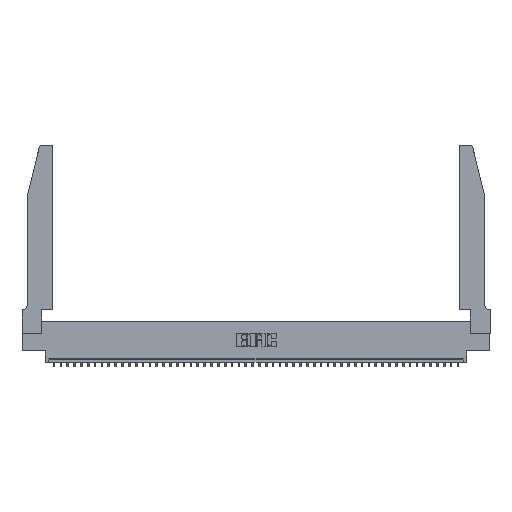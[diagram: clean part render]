
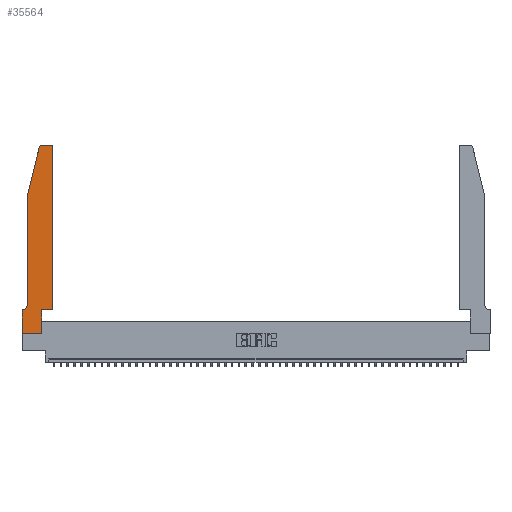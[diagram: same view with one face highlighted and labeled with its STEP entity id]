
A CAD part, top view. The second image highlights one B-rep face of the part: STEP entity #35564.
In plain terms, the highlighted planar face has unit normal (0, 0, 1).
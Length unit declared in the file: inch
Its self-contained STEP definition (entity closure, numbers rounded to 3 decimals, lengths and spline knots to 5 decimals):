
#1839 = CARTESIAN_POINT ( 'NONE',  ( 0.4505, 2.72, 0.37 ) ) ;
#1887 = DIRECTION ( 'NONE',  ( 1., 0., 0. ) ) ;
#2209 = VERTEX_POINT ( 'NONE', #33008 ) ;
#2397 = AXIS2_PLACEMENT_3D ( 'NONE', #25346, #14552, #6997 ) ;
#2660 = DIRECTION ( 'NONE',  ( 0., -1., 0. ) ) ;
#3910 = DIRECTION ( 'NONE',  ( 0., -1., 0. ) ) ;
#4577 = DIRECTION ( 'NONE',  ( 0., 1., 0. ) ) ;
#4760 = CARTESIAN_POINT ( 'NONE',  ( 0.2865, 0.35, 0.37 ) ) ;
#4791 = AXIS2_PLACEMENT_3D ( 'NONE', #44145, #21708, #29166 ) ;
#4852 = CARTESIAN_POINT ( 'NONE',  ( 0.2865, 0.35, 0.37 ) ) ;
#5420 = ORIENTED_EDGE ( 'NONE', *, *, #15437, .T. ) ;
#5461 = EDGE_CURVE ( 'NONE', #43064, #2209, #45747, .T. ) ;
#6198 = CIRCLE ( 'NONE', #37519, 0.03 ) ;
#6532 = CARTESIAN_POINT ( 'NONE',  ( 0.0755, 2., 0.37 ) ) ;
#6580 = LINE ( 'NONE', #20166, #33542 ) ;
#6997 = DIRECTION ( 'NONE',  ( 1., 0., 0. ) ) ;
#7316 = AXIS2_PLACEMENT_3D ( 'NONE', #16678, #38601, #20360 ) ;
#7540 = ORIENTED_EDGE ( 'NONE', *, *, #13173, .T. ) ;
#8031 = CARTESIAN_POINT ( 'NONE',  ( 0.0055, 0.35, 0.37 ) ) ;
#8186 = VECTOR ( 'NONE', #8944, 39.37008 ) ;
#8944 = DIRECTION ( 'NONE',  ( 1., 0., 0. ) ) ;
#11055 = EDGE_CURVE ( 'NONE', #25771, #43064, #26570, .T. ) ;
#12054 = VECTOR ( 'NONE', #23379, 39.37008 ) ;
#13173 = EDGE_CURVE ( 'NONE', #31391, #26869, #25869, .T. ) ;
#13547 = CARTESIAN_POINT ( 'NONE',  ( 0.284, 2.75, 0.37 ) ) ;
#13766 = ORIENTED_EDGE ( 'NONE', *, *, #5461, .T. ) ;
#13864 = CARTESIAN_POINT ( 'NONE',  ( 0.4505, 0.35, 0.37 ) ) ;
#14215 = VECTOR ( 'NONE', #4577, 39.37008 ) ;
#14552 = DIRECTION ( 'NONE',  ( 0., 0., 1. ) ) ;
#15160 = VECTOR ( 'NONE', #2660, 39.37008 ) ;
#15437 = EDGE_CURVE ( 'NONE', #26869, #45012, #25602, .T. ) ;
#15613 = ORIENTED_EDGE ( 'NONE', *, *, #32719, .T. ) ;
#16078 = DIRECTION ( 'NONE',  ( 1., 0., 0. ) ) ;
#16669 = ORIENTED_EDGE ( 'NONE', *, *, #11055, .T. ) ;
#16678 = CARTESIAN_POINT ( 'NONE',  ( 0., 0.35, 0.37 ) ) ;
#17177 = EDGE_CURVE ( 'NONE', #21071, #21904, #6580, .T. ) ;
#18057 = CARTESIAN_POINT ( 'NONE',  ( 0.4505, 0.35, 0.37 ) ) ;
#20040 = VECTOR ( 'NONE', #25182, 39.37008 ) ;
#20166 = CARTESIAN_POINT ( 'NONE',  ( 0.2605, 2.75, 0.37 ) ) ;
#20360 = DIRECTION ( 'NONE',  ( 1., 0., 0. ) ) ;
#20470 = LINE ( 'NONE', #4760, #14215 ) ;
#20518 = PLANE ( 'NONE',  #7316 ) ;
#21071 = VERTEX_POINT ( 'NONE', #40611 ) ;
#21300 = EDGE_CURVE ( 'NONE', #26277, #21071, #40802, .T. ) ;
#21496 = CARTESIAN_POINT ( 'NONE',  ( 0., 0., 0.37 ) ) ;
#21708 = DIRECTION ( 'NONE',  ( 0., 0., -1. ) ) ;
#21904 = VERTEX_POINT ( 'NONE', #13547 ) ;
#21989 = EDGE_CURVE ( 'NONE', #21904, #25771, #6198, .T. ) ;
#22930 = VECTOR ( 'NONE', #3910, 39.37008 ) ;
#23076 = VECTOR ( 'NONE', #23717, 39.37008 ) ;
#23379 = DIRECTION ( 'NONE',  ( -1., 0., 0. ) ) ;
#23558 = DIRECTION ( 'NONE',  ( -1., 0., 0. ) ) ;
#23619 = ORIENTED_EDGE ( 'NONE', *, *, #32257, .T. ) ;
#23717 = DIRECTION ( 'NONE',  ( -0.239, -0.971, 0. ) ) ;
#25182 = DIRECTION ( 'NONE',  ( 0., 1., 0. ) ) ;
#25346 = CARTESIAN_POINT ( 'NONE',  ( 0.4205, 2.72, 0.37 ) ) ;
#25602 = LINE ( 'NONE', #41126, #31373 ) ;
#25767 = EDGE_CURVE ( 'NONE', #45012, #26614, #20470, .T. ) ;
#25771 = VERTEX_POINT ( 'NONE', #30188 ) ;
#25869 = LINE ( 'NONE', #43743, #22930 ) ;
#26277 = VERTEX_POINT ( 'NONE', #1839 ) ;
#26570 = LINE ( 'NONE', #34330, #23076 ) ;
#26614 = VERTEX_POINT ( 'NONE', #4852 ) ;
#26829 = VERTEX_POINT ( 'NONE', #13864 ) ;
#26869 = VERTEX_POINT ( 'NONE', #21496 ) ;
#28531 = EDGE_CURVE ( 'NONE', #26614, #26829, #40473, .T. ) ;
#29166 = DIRECTION ( 'NONE',  ( -1., 0., 0. ) ) ;
#29934 = CARTESIAN_POINT ( 'NONE',  ( 0., 0.35, 0.37 ) ) ;
#30188 = CARTESIAN_POINT ( 'NONE',  ( 0.25487, 2.72718, 0.37 ) ) ;
#30238 = EDGE_LOOP ( 'NONE', ( #34583, #45160, #16669, #13766, #40182, #23619, #7540, #5420, #35904, #35687, #15613, #46600 ) ) ;
#30727 = CARTESIAN_POINT ( 'NONE',  ( 0.284, 2.72, 0.37 ) ) ;
#31373 = VECTOR ( 'NONE', #1887, 39.37008 ) ;
#31391 = VERTEX_POINT ( 'NONE', #29934 ) ;
#32257 = EDGE_CURVE ( 'NONE', #32406, #31391, #43799, .T. ) ;
#32406 = VERTEX_POINT ( 'NONE', #8031 ) ;
#32516 = CIRCLE ( 'NONE', #4791, 0.07 ) ;
#32719 = EDGE_CURVE ( 'NONE', #26829, #26277, #34463, .T. ) ;
#33008 = CARTESIAN_POINT ( 'NONE',  ( 0.0755, 0.42, 0.37 ) ) ;
#33542 = VECTOR ( 'NONE', #23558, 39.37008 ) ;
#34330 = CARTESIAN_POINT ( 'NONE',  ( 0.0755, 2., 0.37 ) ) ;
#34463 = LINE ( 'NONE', #18057, #20040 ) ;
#34583 = ORIENTED_EDGE ( 'NONE', *, *, #17177, .T. ) ;
#35564 = ADVANCED_FACE ( 'NONE', ( #46942 ), #20518, .T. ) ;
#35687 = ORIENTED_EDGE ( 'NONE', *, *, #28531, .T. ) ;
#35904 = ORIENTED_EDGE ( 'NONE', *, *, #25767, .T. ) ;
#37519 = AXIS2_PLACEMENT_3D ( 'NONE', #30727, #38147, #16078 ) ;
#38147 = DIRECTION ( 'NONE',  ( 0., 0., 1. ) ) ;
#38601 = DIRECTION ( 'NONE',  ( 0., 0., 1. ) ) ;
#40182 = ORIENTED_EDGE ( 'NONE', *, *, #43640, .T. ) ;
#40473 = LINE ( 'NONE', #42111, #8186 ) ;
#40611 = CARTESIAN_POINT ( 'NONE',  ( 0.4205, 2.75, 0.37 ) ) ;
#40802 = CIRCLE ( 'NONE', #2397, 0.03 ) ;
#41126 = CARTESIAN_POINT ( 'NONE',  ( 0., 0., 0.37 ) ) ;
#41925 = CARTESIAN_POINT ( 'NONE',  ( 0.0755, 0.35, 0.37 ) ) ;
#42111 = CARTESIAN_POINT ( 'NONE',  ( 0.4505, 0.35, 0.37 ) ) ;
#43064 = VERTEX_POINT ( 'NONE', #6532 ) ;
#43640 = EDGE_CURVE ( 'NONE', #2209, #32406, #32516, .T. ) ;
#43743 = CARTESIAN_POINT ( 'NONE',  ( 0., 0., 0.37 ) ) ;
#43799 = LINE ( 'NONE', #41925, #12054 ) ;
#43972 = CARTESIAN_POINT ( 'NONE',  ( 0.2865, 0., 0.37 ) ) ;
#44145 = CARTESIAN_POINT ( 'NONE',  ( 0.0055, 0.42, 0.37 ) ) ;
#45012 = VERTEX_POINT ( 'NONE', #43972 ) ;
#45160 = ORIENTED_EDGE ( 'NONE', *, *, #21989, .T. ) ;
#45747 = LINE ( 'NONE', #46480, #15160 ) ;
#46480 = CARTESIAN_POINT ( 'NONE',  ( 0.0755, 2., 0.37 ) ) ;
#46600 = ORIENTED_EDGE ( 'NONE', *, *, #21300, .T. ) ;
#46942 = FACE_OUTER_BOUND ( 'NONE', #30238, .T. ) ;
